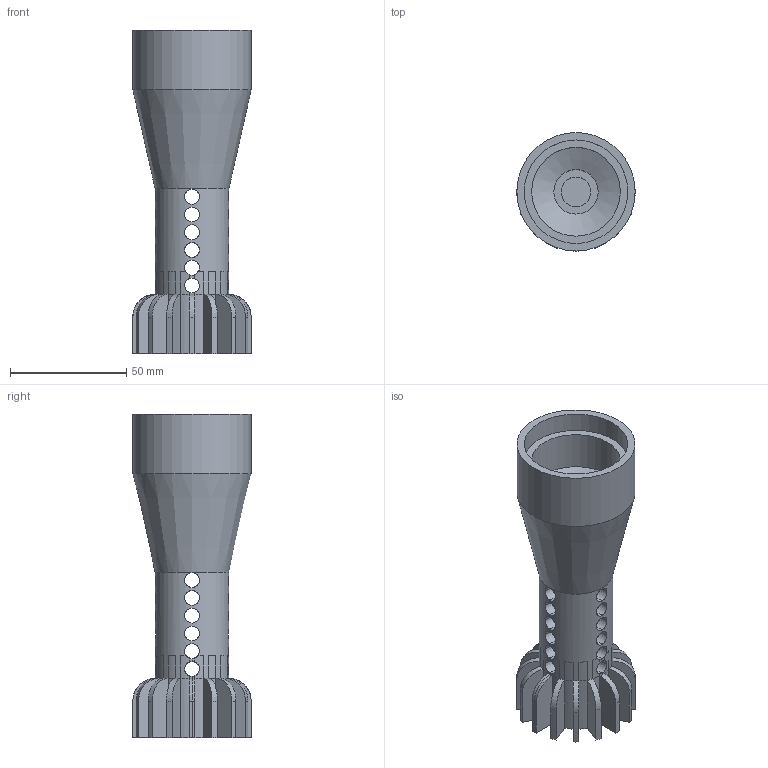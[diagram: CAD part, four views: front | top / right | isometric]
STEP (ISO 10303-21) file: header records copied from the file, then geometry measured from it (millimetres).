
FILE_DESCRIPTION(('Open CASCADE Model'),'2;1');
FILE_NAME('Open CASCADE Shape Model','2013-06-16T13:40:48',('Author'),( 'Open CASCADE'),'Open CASCADE STEP processor 6.1','Open CASCADE 6.1' ,'Unknown');
FILE_SCHEMA(('AUTOMOTIVE_DESIGN_CC2 { 1 2 10303 214 -1 1 5 4 }'));
Length unit declared in the file: millimetre
Products named in the file (1): Product 1
Bounding box: 50.8 x 50.8 x 138.68 mm (x, y, z)
Volume: 106389.6 mm3; surface area: 37650.3 mm2
Topology: 1 solids, 1 shells, 219 faces, 655 edges, 424 vertices
Faces by surface type: bspline 144, cylinder 50, torus 17, plane 6, cone 2
Full cylindrical faces by diameter (mm): 12.7 x1, 19.05 x1, 20.345 x1, 31.75 x1, 38.1 x1, 44.45 x1, 50.8 x1
Entity records: 191406 total; most frequent: CARTESIAN_POINT 181540, B_SPLINE_CURVE_WITH_KNOTS 1400, ORIENTED_EDGE 1310, PCURVE 1310, DEFINITIONAL_REPRESENTATION 1310, DIRECTION 782, EDGE_CURVE 655, SURFACE_CURVE 636
